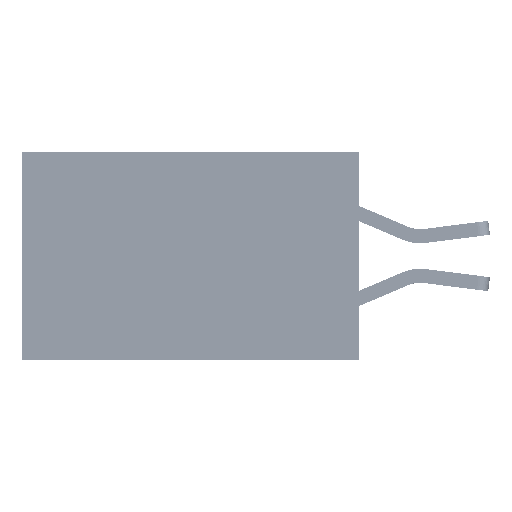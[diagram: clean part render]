
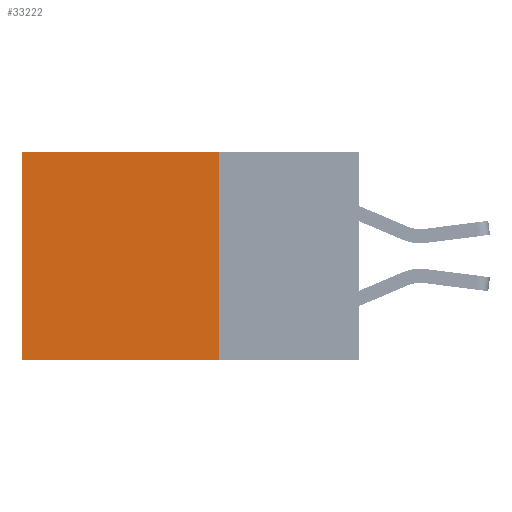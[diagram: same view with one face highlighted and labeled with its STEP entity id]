
A CAD part, left-side view. The second image highlights one B-rep face of the part: STEP entity #33222.
In plain terms, the highlighted planar face has unit normal (-1, 0, 0).
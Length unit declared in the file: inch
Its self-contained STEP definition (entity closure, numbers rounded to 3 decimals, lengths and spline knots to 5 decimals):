
#262 = DIRECTION ( 'NONE',  ( 0., 0., -1. ) ) ;
#725 = ORIENTED_EDGE ( 'NONE', *, *, #47140, .T. ) ;
#1324 = CARTESIAN_POINT ( 'NONE',  ( 0.2875, 0.25, -0.37 ) ) ;
#1561 = LINE ( 'NONE', #29861, #29679 ) ;
#6732 = VERTEX_POINT ( 'NONE', #18344 ) ;
#8144 = CARTESIAN_POINT ( 'NONE',  ( 0.2875, 0.6, -0.37 ) ) ;
#8733 = EDGE_CURVE ( 'NONE', #16054, #17123, #44031, .T. ) ;
#9181 = EDGE_CURVE ( 'NONE', #17123, #27073, #21381, .T. ) ;
#9656 = CARTESIAN_POINT ( 'NONE',  ( 0.2875, 0.6, 0. ) ) ;
#10960 = DIRECTION ( 'NONE',  ( 0., 0., -1. ) ) ;
#15112 = EDGE_LOOP ( 'NONE', ( #47159, #46012, #18231, #725 ) ) ;
#15677 = EDGE_CURVE ( 'NONE', #6732, #27073, #32213, .T. ) ;
#16054 = VERTEX_POINT ( 'NONE', #27078 ) ;
#17123 = VERTEX_POINT ( 'NONE', #46539 ) ;
#17292 = AXIS2_PLACEMENT_3D ( 'NONE', #19379, #26688, #262 ) ;
#18231 = ORIENTED_EDGE ( 'NONE', *, *, #8733, .F. ) ;
#18344 = CARTESIAN_POINT ( 'NONE',  ( 0.2875, 0.6, 0. ) ) ;
#19379 = CARTESIAN_POINT ( 'NONE',  ( 0.2875, 0.25, 0. ) ) ;
#21381 = LINE ( 'NONE', #1324, #42819 ) ;
#24814 = DIRECTION ( 'NONE',  ( 0., 0., -1. ) ) ;
#26688 = DIRECTION ( 'NONE',  ( 1., 0., 0. ) ) ;
#27073 = VERTEX_POINT ( 'NONE', #8144 ) ;
#27078 = CARTESIAN_POINT ( 'NONE',  ( 0.2875, 0.25, 0. ) ) ;
#28083 = DIRECTION ( 'NONE',  ( 0., 1., 0. ) ) ;
#29402 = FACE_OUTER_BOUND ( 'NONE', #15112, .T. ) ;
#29679 = VECTOR ( 'NONE', #49303, 39.37008 ) ;
#29861 = CARTESIAN_POINT ( 'NONE',  ( 0.2875, 0.25, 0. ) ) ;
#32213 = LINE ( 'NONE', #9656, #45896 ) ;
#33222 = ADVANCED_FACE ( 'NONE', ( #29402 ), #38327, .F. ) ;
#38327 = PLANE ( 'NONE',  #17292 ) ;
#41061 = VECTOR ( 'NONE', #10960, 39.37008 ) ;
#42819 = VECTOR ( 'NONE', #28083, 39.37008 ) ;
#44031 = LINE ( 'NONE', #48761, #41061 ) ;
#45896 = VECTOR ( 'NONE', #24814, 39.37008 ) ;
#46012 = ORIENTED_EDGE ( 'NONE', *, *, #9181, .F. ) ;
#46539 = CARTESIAN_POINT ( 'NONE',  ( 0.2875, 0.25, -0.37 ) ) ;
#47140 = EDGE_CURVE ( 'NONE', #16054, #6732, #1561, .T. ) ;
#47159 = ORIENTED_EDGE ( 'NONE', *, *, #15677, .T. ) ;
#48761 = CARTESIAN_POINT ( 'NONE',  ( 0.2875, 0.25, 0. ) ) ;
#49303 = DIRECTION ( 'NONE',  ( 0., 1., 0. ) ) ;
